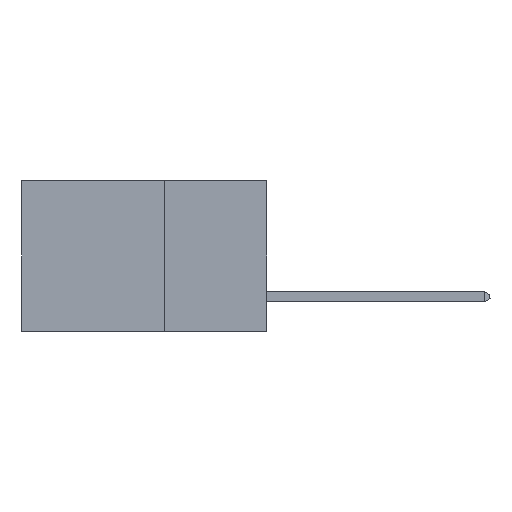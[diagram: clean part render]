
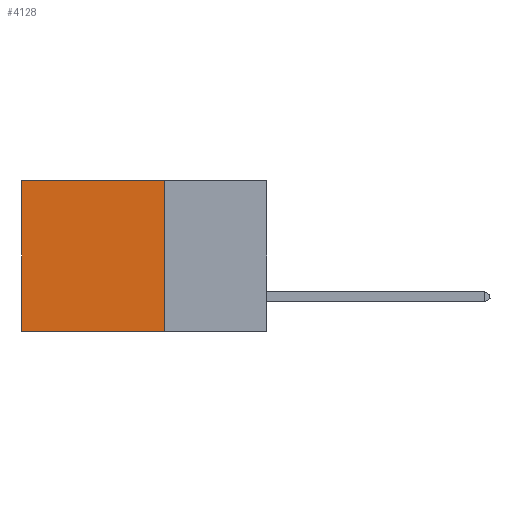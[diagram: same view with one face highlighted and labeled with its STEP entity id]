
A CAD part, left-side view. The second image highlights one B-rep face of the part: STEP entity #4128.
In plain terms, the highlighted planar face has unit normal (-1, 0, 0).
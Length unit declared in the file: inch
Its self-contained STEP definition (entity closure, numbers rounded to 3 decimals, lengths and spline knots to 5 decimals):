
#31 = AXIS2_PLACEMENT_3D ( 'NONE', #17743, #2277, #7425 ) ;
#663 = DIRECTION ( 'NONE',  ( 0., 0., -1. ) ) ;
#756 = VECTOR ( 'NONE', #21833, 39.37008 ) ;
#1168 = EDGE_CURVE ( 'NONE', #20481, #17155, #10987, .T. ) ;
#1316 = DIRECTION ( 'NONE',  ( 0., 1., 0. ) ) ;
#1419 = ORIENTED_EDGE ( 'NONE', *, *, #1997, .T. ) ;
#1656 = EDGE_CURVE ( 'NONE', #21495, #17155, #19569, .T. ) ;
#1997 = EDGE_CURVE ( 'NONE', #16394, #21495, #8532, .T. ) ;
#2277 = DIRECTION ( 'NONE',  ( 1., 0., 0. ) ) ;
#2742 = ORIENTED_EDGE ( 'NONE', *, *, #1168, .F. ) ;
#4128 = ADVANCED_FACE ( 'NONE', ( #5026 ), #7195, .F. ) ;
#4289 = ORIENTED_EDGE ( 'NONE', *, *, #18558, .F. ) ;
#5026 = FACE_OUTER_BOUND ( 'NONE', #16600, .T. ) ;
#6843 = CARTESIAN_POINT ( 'NONE',  ( 0.2875, 0.25, -0.37 ) ) ;
#7195 = PLANE ( 'NONE',  #31 ) ;
#7425 = DIRECTION ( 'NONE',  ( 0., 0., -1. ) ) ;
#7441 = CARTESIAN_POINT ( 'NONE',  ( 0.2875, 0.25, 0. ) ) ;
#8532 = LINE ( 'NONE', #7441, #14699 ) ;
#10987 = LINE ( 'NONE', #21923, #13416 ) ;
#12043 = CARTESIAN_POINT ( 'NONE',  ( 0.2875, 0.6, 0. ) ) ;
#12783 = VECTOR ( 'NONE', #663, 39.37008 ) ;
#13072 = LINE ( 'NONE', #15902, #12783 ) ;
#13073 = CARTESIAN_POINT ( 'NONE',  ( 0.2875, 0.6, 0. ) ) ;
#13416 = VECTOR ( 'NONE', #1316, 39.37008 ) ;
#14699 = VECTOR ( 'NONE', #15937, 39.37008 ) ;
#15202 = CARTESIAN_POINT ( 'NONE',  ( 0.2875, 0.6, -0.37 ) ) ;
#15368 = ORIENTED_EDGE ( 'NONE', *, *, #1656, .T. ) ;
#15902 = CARTESIAN_POINT ( 'NONE',  ( 0.2875, 0.25, 0. ) ) ;
#15937 = DIRECTION ( 'NONE',  ( 0., 1., 0. ) ) ;
#16394 = VERTEX_POINT ( 'NONE', #18748 ) ;
#16600 = EDGE_LOOP ( 'NONE', ( #15368, #2742, #4289, #1419 ) ) ;
#17155 = VERTEX_POINT ( 'NONE', #15202 ) ;
#17743 = CARTESIAN_POINT ( 'NONE',  ( 0.2875, 0.25, 0. ) ) ;
#18558 = EDGE_CURVE ( 'NONE', #16394, #20481, #13072, .T. ) ;
#18748 = CARTESIAN_POINT ( 'NONE',  ( 0.2875, 0.25, 0. ) ) ;
#19569 = LINE ( 'NONE', #13073, #756 ) ;
#20481 = VERTEX_POINT ( 'NONE', #6843 ) ;
#21495 = VERTEX_POINT ( 'NONE', #12043 ) ;
#21833 = DIRECTION ( 'NONE',  ( 0., 0., -1. ) ) ;
#21923 = CARTESIAN_POINT ( 'NONE',  ( 0.2875, 0.25, -0.37 ) ) ;
